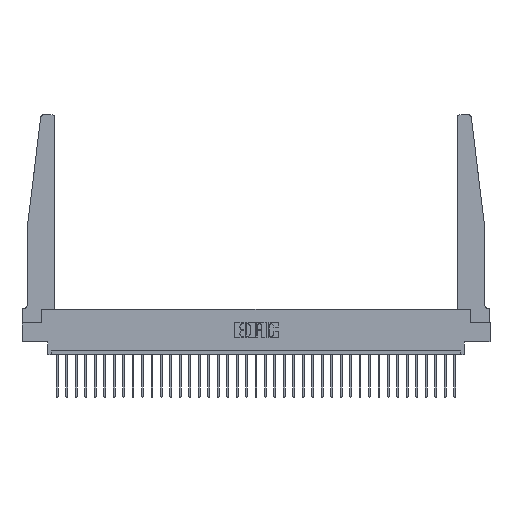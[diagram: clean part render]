
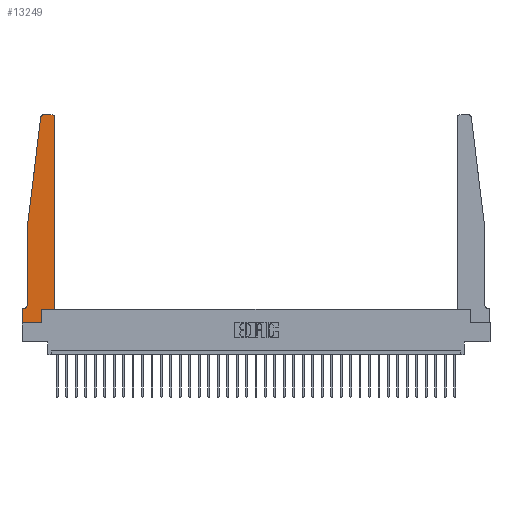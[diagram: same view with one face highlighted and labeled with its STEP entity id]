
A CAD part, top view. The second image highlights one B-rep face of the part: STEP entity #13249.
In plain terms, the highlighted planar face has unit normal (0, 0, 1).
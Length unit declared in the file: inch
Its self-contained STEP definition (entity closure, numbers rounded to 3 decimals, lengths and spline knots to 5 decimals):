
#319 = CARTESIAN_POINT ( 'NONE',  ( 0.065, 0.2375, 0.37 ) ) ;
#577 = CARTESIAN_POINT ( 'NONE',  ( 0.24675, 2.72367, 0.37 ) ) ;
#834 = VERTEX_POINT ( 'NONE', #3517 ) ;
#1215 = LINE ( 'NONE', #26056, #16110 ) ;
#1645 = DIRECTION ( 'NONE',  ( 0., -1., 0. ) ) ;
#1675 = VECTOR ( 'NONE', #13595, 39.37008 ) ;
#2064 = EDGE_CURVE ( 'NONE', #20952, #9994, #6887, .T. ) ;
#2938 = VERTEX_POINT ( 'NONE', #28866 ) ;
#3203 = DIRECTION ( 'NONE',  ( -1., 0., 0. ) ) ;
#3517 = CARTESIAN_POINT ( 'NONE',  ( 0.2605, 0., 0.37 ) ) ;
#3632 = VECTOR ( 'NONE', #30525, 39.37008 ) ;
#3682 = DIRECTION ( 'NONE',  ( 0., 0., -1. ) ) ;
#3783 = ORIENTED_EDGE ( 'NONE', *, *, #9392, .T. ) ;
#4017 = DIRECTION ( 'NONE',  ( 1., 0., 0. ) ) ;
#4640 = CARTESIAN_POINT ( 'NONE',  ( 0.425, 0.18, 0.37 ) ) ;
#4853 = LINE ( 'NONE', #16495, #18536 ) ;
#5184 = VECTOR ( 'NONE', #19561, 39.37008 ) ;
#5453 = ORIENTED_EDGE ( 'NONE', *, *, #9612, .T. ) ;
#5750 = AXIS2_PLACEMENT_3D ( 'NONE', #30966, #8840, #4017 ) ;
#5774 = EDGE_CURVE ( 'NONE', #26226, #21489, #4853, .T. ) ;
#5787 = AXIS2_PLACEMENT_3D ( 'NONE', #30837, #28883, #16626 ) ;
#5835 = VECTOR ( 'NONE', #9728, 39.37008 ) ;
#6165 = CARTESIAN_POINT ( 'NONE',  ( 0.25, 2.75, 0.37 ) ) ;
#6887 = LINE ( 'NONE', #4640, #9409 ) ;
#7059 = ORIENTED_EDGE ( 'NONE', *, *, #10337, .T. ) ;
#7141 = CARTESIAN_POINT ( 'NONE',  ( 0., 0., 0.37 ) ) ;
#7448 = ORIENTED_EDGE ( 'NONE', *, *, #5774, .T. ) ;
#7514 = VERTEX_POINT ( 'NONE', #7816 ) ;
#7816 = CARTESIAN_POINT ( 'NONE',  ( 0.425, 2.72, 0.37 ) ) ;
#8078 = EDGE_LOOP ( 'NONE', ( #3783, #15284, #12312, #7448, #31301, #31422, #11849, #24005, #22178, #11754, #7059, #5453 ) ) ;
#8131 = CARTESIAN_POINT ( 'NONE',  ( 0.395, 2.75, 0.37 ) ) ;
#8840 = DIRECTION ( 'NONE',  ( 0., 0., 1. ) ) ;
#9157 = PLANE ( 'NONE',  #20392 ) ;
#9392 = EDGE_CURVE ( 'NONE', #20756, #12971, #19240, .T. ) ;
#9409 = VECTOR ( 'NONE', #14480, 39.37008 ) ;
#9474 = DIRECTION ( 'NONE',  ( 0., -1., 0. ) ) ;
#9612 = EDGE_CURVE ( 'NONE', #7514, #20756, #15079, .T. ) ;
#9728 = DIRECTION ( 'NONE',  ( 1., 0., 0. ) ) ;
#9994 = VERTEX_POINT ( 'NONE', #28039 ) ;
#10250 = CARTESIAN_POINT ( 'NONE',  ( 0., 0.1875, 0.37 ) ) ;
#10337 = EDGE_CURVE ( 'NONE', #9994, #7514, #1215, .T. ) ;
#10500 = VECTOR ( 'NONE', #10914, 39.37008 ) ;
#10599 = EDGE_CURVE ( 'NONE', #26840, #834, #19421, .T. ) ;
#10914 = DIRECTION ( 'NONE',  ( -0.122, -0.992, 0. ) ) ;
#11045 = DIRECTION ( 'NONE',  ( 0., 1., 0. ) ) ;
#11754 = ORIENTED_EDGE ( 'NONE', *, *, #2064, .T. ) ;
#11787 = EDGE_CURVE ( 'NONE', #18608, #26226, #15623, .T. ) ;
#11849 = ORIENTED_EDGE ( 'NONE', *, *, #27814, .T. ) ;
#12312 = ORIENTED_EDGE ( 'NONE', *, *, #11787, .T. ) ;
#12971 = VERTEX_POINT ( 'NONE', #19664 ) ;
#13249 = ADVANCED_FACE ( 'NONE', ( #31278 ), #9157, .T. ) ;
#13322 = CARTESIAN_POINT ( 'NONE',  ( 0., 0., 0.37 ) ) ;
#13431 = VERTEX_POINT ( 'NONE', #10250 ) ;
#13595 = DIRECTION ( 'NONE',  ( -1., 0., 0. ) ) ;
#14480 = DIRECTION ( 'NONE',  ( 1., 0., 0. ) ) ;
#15079 = CIRCLE ( 'NONE', #5787, 0.03 ) ;
#15284 = ORIENTED_EDGE ( 'NONE', *, *, #22718, .T. ) ;
#15623 = LINE ( 'NONE', #18048, #10500 ) ;
#16110 = VECTOR ( 'NONE', #11045, 39.37008 ) ;
#16495 = CARTESIAN_POINT ( 'NONE',  ( 0.065, 1.25, 0.37 ) ) ;
#16626 = DIRECTION ( 'NONE',  ( 1., 0., 0. ) ) ;
#16745 = DIRECTION ( 'NONE',  ( 1., 0., 0. ) ) ;
#18048 = CARTESIAN_POINT ( 'NONE',  ( 0.065, 1.25, 0.37 ) ) ;
#18536 = VECTOR ( 'NONE', #1645, 39.37008 ) ;
#18608 = VERTEX_POINT ( 'NONE', #577 ) ;
#18619 = CARTESIAN_POINT ( 'NONE',  ( 0.2605, 0.18, 0.37 ) ) ;
#19014 = DIRECTION ( 'NONE',  ( 0., 0., 1. ) ) ;
#19240 = LINE ( 'NONE', #6165, #1675 ) ;
#19421 = LINE ( 'NONE', #7141, #5835 ) ;
#19561 = DIRECTION ( 'NONE',  ( 0., 1., 0. ) ) ;
#19664 = CARTESIAN_POINT ( 'NONE',  ( 0.27653, 2.75, 0.37 ) ) ;
#19719 = LINE ( 'NONE', #29091, #5184 ) ;
#20392 = AXIS2_PLACEMENT_3D ( 'NONE', #24292, #19014, #16745 ) ;
#20756 = VERTEX_POINT ( 'NONE', #8131 ) ;
#20952 = VERTEX_POINT ( 'NONE', #18619 ) ;
#21105 = EDGE_CURVE ( 'NONE', #834, #20952, #19719, .T. ) ;
#21221 = EDGE_CURVE ( 'NONE', #2938, #13431, #23088, .T. ) ;
#21489 = VERTEX_POINT ( 'NONE', #319 ) ;
#22178 = ORIENTED_EDGE ( 'NONE', *, *, #21105, .T. ) ;
#22609 = EDGE_CURVE ( 'NONE', #21489, #2938, #23780, .T. ) ;
#22718 = EDGE_CURVE ( 'NONE', #12971, #18608, #29989, .T. ) ;
#23088 = LINE ( 'NONE', #28408, #3632 ) ;
#23780 = CIRCLE ( 'NONE', #24298, 0.05 ) ;
#24005 = ORIENTED_EDGE ( 'NONE', *, *, #10599, .T. ) ;
#24086 = CARTESIAN_POINT ( 'NONE',  ( 0.065, 1.25, 0.37 ) ) ;
#24292 = CARTESIAN_POINT ( 'NONE',  ( 0., 0.1875, 0.37 ) ) ;
#24298 = AXIS2_PLACEMENT_3D ( 'NONE', #25781, #3682, #3203 ) ;
#25781 = CARTESIAN_POINT ( 'NONE',  ( 0.015, 0.2375, 0.37 ) ) ;
#26056 = CARTESIAN_POINT ( 'NONE',  ( 0.425, 0.18, 0.37 ) ) ;
#26226 = VERTEX_POINT ( 'NONE', #24086 ) ;
#26840 = VERTEX_POINT ( 'NONE', #13322 ) ;
#27040 = VECTOR ( 'NONE', #9474, 39.37008 ) ;
#27814 = EDGE_CURVE ( 'NONE', #13431, #26840, #29483, .T. ) ;
#28039 = CARTESIAN_POINT ( 'NONE',  ( 0.425, 0.18, 0.37 ) ) ;
#28408 = CARTESIAN_POINT ( 'NONE',  ( 0.065, 0.1875, 0.37 ) ) ;
#28866 = CARTESIAN_POINT ( 'NONE',  ( 0.015, 0.1875, 0.37 ) ) ;
#28883 = DIRECTION ( 'NONE',  ( 0., 0., 1. ) ) ;
#29091 = CARTESIAN_POINT ( 'NONE',  ( 0.2605, 0.18, 0.37 ) ) ;
#29330 = CARTESIAN_POINT ( 'NONE',  ( 0., 0., 0.37 ) ) ;
#29483 = LINE ( 'NONE', #29330, #27040 ) ;
#29989 = CIRCLE ( 'NONE', #5750, 0.03 ) ;
#30525 = DIRECTION ( 'NONE',  ( -1., 0., 0. ) ) ;
#30837 = CARTESIAN_POINT ( 'NONE',  ( 0.395, 2.72, 0.37 ) ) ;
#30966 = CARTESIAN_POINT ( 'NONE',  ( 0.27653, 2.72, 0.37 ) ) ;
#31278 = FACE_OUTER_BOUND ( 'NONE', #8078, .T. ) ;
#31301 = ORIENTED_EDGE ( 'NONE', *, *, #22609, .T. ) ;
#31422 = ORIENTED_EDGE ( 'NONE', *, *, #21221, .T. ) ;
